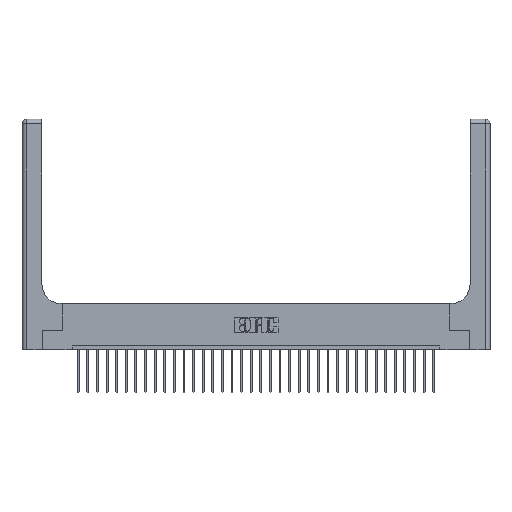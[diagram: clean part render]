
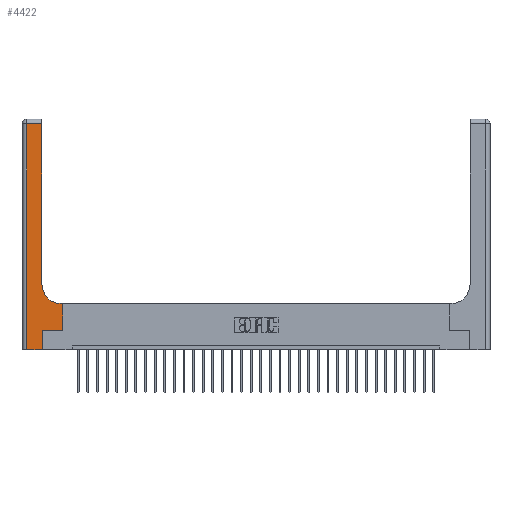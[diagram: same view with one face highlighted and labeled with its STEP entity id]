
A CAD part, top view. The second image highlights one B-rep face of the part: STEP entity #4422.
In plain terms, the highlighted planar face has unit normal (0, 0, 1).
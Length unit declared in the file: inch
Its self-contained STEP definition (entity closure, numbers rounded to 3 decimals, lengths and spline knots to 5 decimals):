
#113 = EDGE_CURVE ( 'NONE', #22762, #16638, #9215, .T. ) ;
#248 = DIRECTION ( 'NONE',  ( 0., 1., 0. ) ) ;
#619 = ORIENTED_EDGE ( 'NONE', *, *, #2468, .T. ) ;
#731 = CARTESIAN_POINT ( 'NONE',  ( 0., 3., 0.37 ) ) ;
#885 = CARTESIAN_POINT ( 'NONE',  ( 0.265, 0.25, 0.37 ) ) ;
#1218 = CARTESIAN_POINT ( 'NONE',  ( 0.528, 0.25, 0.37 ) ) ;
#2468 = EDGE_CURVE ( 'NONE', #3541, #20409, #18991, .T. ) ;
#2730 = CARTESIAN_POINT ( 'NONE',  ( 0.528, 0.25, 0.37 ) ) ;
#3072 = ORIENTED_EDGE ( 'NONE', *, *, #7748, .T. ) ;
#3541 = VERTEX_POINT ( 'NONE', #16745 ) ;
#4392 = LINE ( 'NONE', #12727, #7621 ) ;
#4422 = ADVANCED_FACE ( 'NONE', ( #7706 ), #5060, .F. ) ;
#4625 = LINE ( 'NONE', #15554, #21318 ) ;
#4816 = AXIS2_PLACEMENT_3D ( 'NONE', #26472, #17617, #10907 ) ;
#4960 = CARTESIAN_POINT ( 'NONE',  ( 0.265, 0.25, 0.37 ) ) ;
#5060 = PLANE ( 'NONE',  #22870 ) ;
#5363 = DIRECTION ( 'NONE',  ( 0., 1., 0. ) ) ;
#5446 = VECTOR ( 'NONE', #20996, 39.37008 ) ;
#5534 = VERTEX_POINT ( 'NONE', #19932 ) ;
#6222 = VECTOR ( 'NONE', #19809, 39.37008 ) ;
#6418 = DIRECTION ( 'NONE',  ( 0., -1., 0. ) ) ;
#6526 = CARTESIAN_POINT ( 'NONE',  ( 0.26, 0.85, 0.37 ) ) ;
#7262 = DIRECTION ( 'NONE',  ( 1., 0., 0. ) ) ;
#7621 = VECTOR ( 'NONE', #19563, 39.37008 ) ;
#7706 = FACE_OUTER_BOUND ( 'NONE', #13189, .T. ) ;
#7748 = EDGE_CURVE ( 'NONE', #23378, #28376, #19240, .T. ) ;
#9067 = VECTOR ( 'NONE', #248, 39.37008 ) ;
#9215 = LINE ( 'NONE', #19050, #20896 ) ;
#9332 = EDGE_CURVE ( 'NONE', #20409, #23378, #25100, .T. ) ;
#9828 = CARTESIAN_POINT ( 'NONE',  ( 0.06, 2.94, 0.37 ) ) ;
#10344 = VERTEX_POINT ( 'NONE', #9828 ) ;
#10907 = DIRECTION ( 'NONE',  ( 1., 0., 0. ) ) ;
#10989 = VECTOR ( 'NONE', #7262, 39.37008 ) ;
#11466 = VERTEX_POINT ( 'NONE', #2730 ) ;
#11818 = DIRECTION ( 'NONE',  ( 0., 1., 0. ) ) ;
#12291 = ORIENTED_EDGE ( 'NONE', *, *, #113, .T. ) ;
#12727 = CARTESIAN_POINT ( 'NONE',  ( 0., 2.94, 0.37 ) ) ;
#13189 = EDGE_LOOP ( 'NONE', ( #3072, #24366, #20548, #20612, #12291, #21759, #26320, #619, #13934 ) ) ;
#13934 = ORIENTED_EDGE ( 'NONE', *, *, #9332, .T. ) ;
#14135 = DIRECTION ( 'NONE',  ( -1., 0., 0. ) ) ;
#14138 = CARTESIAN_POINT ( 'NONE',  ( 0.26, 2.94, 0.37 ) ) ;
#15554 = CARTESIAN_POINT ( 'NONE',  ( 0.06, 3., 0.37 ) ) ;
#16167 = LINE ( 'NONE', #1218, #9067 ) ;
#16638 = VERTEX_POINT ( 'NONE', #885 ) ;
#16745 = CARTESIAN_POINT ( 'NONE',  ( 0.528, 0.6, 0.37 ) ) ;
#17617 = DIRECTION ( 'NONE',  ( 0., 0., -1. ) ) ;
#17653 = EDGE_CURVE ( 'NONE', #10344, #5534, #4625, .T. ) ;
#18596 = EDGE_CURVE ( 'NONE', #16638, #11466, #23725, .T. ) ;
#18835 = DIRECTION ( 'NONE',  ( 0., 0., -1. ) ) ;
#18954 = CARTESIAN_POINT ( 'NONE',  ( 0.51, 0.6, 0.37 ) ) ;
#18991 = LINE ( 'NONE', #24931, #6222 ) ;
#19050 = CARTESIAN_POINT ( 'NONE',  ( 0.265, 0., 0.37 ) ) ;
#19240 = LINE ( 'NONE', #20934, #25546 ) ;
#19563 = DIRECTION ( 'NONE',  ( -1., 0., 0. ) ) ;
#19809 = DIRECTION ( 'NONE',  ( -1., 0., 0. ) ) ;
#19932 = CARTESIAN_POINT ( 'NONE',  ( 0.06, 0., 0.37 ) ) ;
#20409 = VERTEX_POINT ( 'NONE', #18954 ) ;
#20548 = ORIENTED_EDGE ( 'NONE', *, *, #17653, .T. ) ;
#20612 = ORIENTED_EDGE ( 'NONE', *, *, #25330, .T. ) ;
#20892 = EDGE_CURVE ( 'NONE', #11466, #3541, #16167, .T. ) ;
#20896 = VECTOR ( 'NONE', #5363, 39.37008 ) ;
#20934 = CARTESIAN_POINT ( 'NONE',  ( 0.26, 3., 0.37 ) ) ;
#20996 = DIRECTION ( 'NONE',  ( 1., 0., 0. ) ) ;
#21021 = CARTESIAN_POINT ( 'NONE',  ( 0.265, 0., 0.37 ) ) ;
#21090 = CARTESIAN_POINT ( 'NONE',  ( 0., 0., 0.37 ) ) ;
#21318 = VECTOR ( 'NONE', #6418, 39.37008 ) ;
#21759 = ORIENTED_EDGE ( 'NONE', *, *, #18596, .T. ) ;
#22475 = LINE ( 'NONE', #21090, #5446 ) ;
#22762 = VERTEX_POINT ( 'NONE', #21021 ) ;
#22870 = AXIS2_PLACEMENT_3D ( 'NONE', #731, #18835, #14135 ) ;
#23378 = VERTEX_POINT ( 'NONE', #6526 ) ;
#23725 = LINE ( 'NONE', #4960, #10989 ) ;
#24366 = ORIENTED_EDGE ( 'NONE', *, *, #24980, .T. ) ;
#24931 = CARTESIAN_POINT ( 'NONE',  ( 0.26, 0.6, 0.37 ) ) ;
#24980 = EDGE_CURVE ( 'NONE', #28376, #10344, #4392, .T. ) ;
#25100 = CIRCLE ( 'NONE', #4816, 0.25 ) ;
#25330 = EDGE_CURVE ( 'NONE', #5534, #22762, #22475, .T. ) ;
#25546 = VECTOR ( 'NONE', #11818, 39.37008 ) ;
#26320 = ORIENTED_EDGE ( 'NONE', *, *, #20892, .T. ) ;
#26472 = CARTESIAN_POINT ( 'NONE',  ( 0.51, 0.85, 0.37 ) ) ;
#28376 = VERTEX_POINT ( 'NONE', #14138 ) ;
